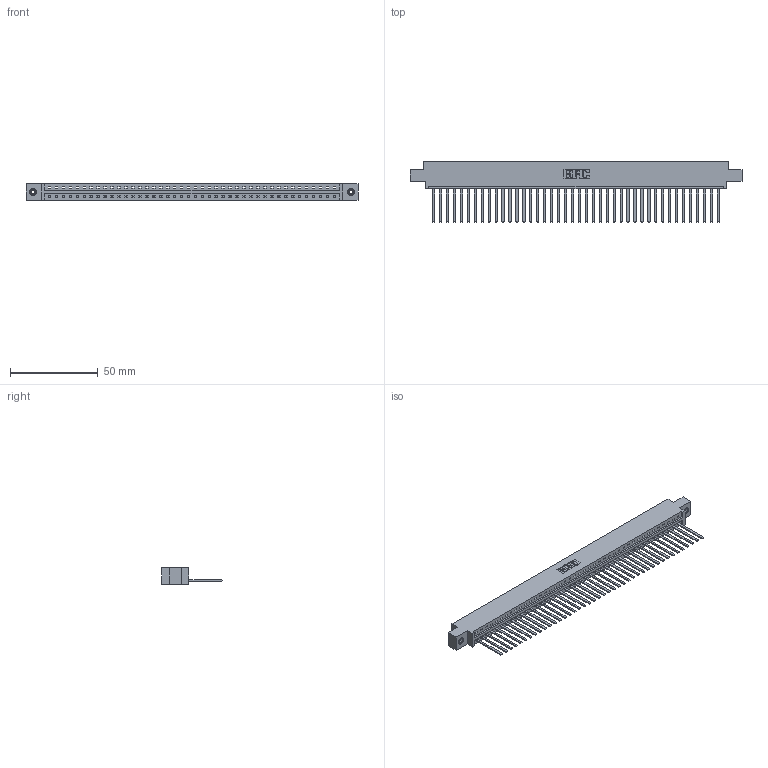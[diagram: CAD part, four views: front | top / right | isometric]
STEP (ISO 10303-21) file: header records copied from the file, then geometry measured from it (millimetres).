
FILE_DESCRIPTION (( 'STEP AP203' ), '1' );
FILE_NAME ('387-042-544-608.STEP', '2018-09-19T23:13:31', ( '' ), ( '' ), 'SwSTEP 2.0', 'SolidWorks 2016', '' );
FILE_SCHEMA (( 'CONFIG_CONTROL_DESIGN' ));
Length unit declared in the file: inch
Products named in the file (4): 345-250-001_345-250-003-102; 387-042-544-608; 337 Part_0.170 Offset - 0.156 Dia-TI; 345-292-001_345-293-144
Assembly tree (45 placements, depth 2):
  387-042-544-608
    337 Part_0.170 Offset - 0.156 Dia-TI
    345-292-001_345-293-144  x42
    345-250-001_345-250-003-102  x2
Bounding box: 189.43 x 34.3 x 9.4 mm (x, y, z)
Volume: 20050.8 mm3; surface area: 22445.8 mm2
Topology: 45 solids, 45 shells, 2530 faces, 7599 edges, 5002 vertices
Faces by surface type: plane 1870, cylinder 644, cone 12, torus 4
Entity records: 32354 total; most frequent: CARTESIAN_POINT 5615, ORIENTED_EDGE 5586, DIRECTION 4755, EDGE_CURVE 2793, VECTOR 2649, LINE 2649, VERTEX_POINT 1856, AXIS2_PLACEMENT_3D 1053
